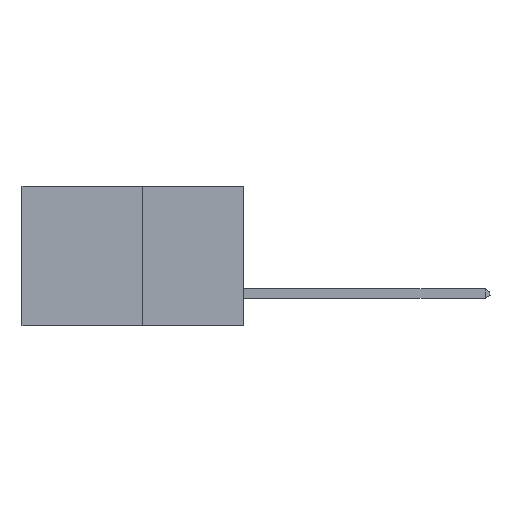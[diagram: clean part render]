
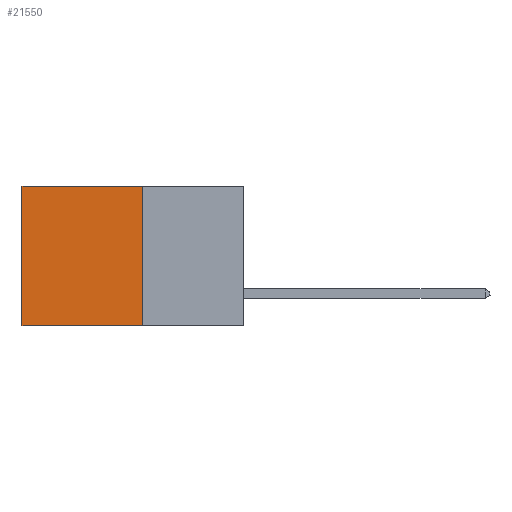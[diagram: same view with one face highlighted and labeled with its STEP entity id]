
A CAD part, left-side view. The second image highlights one B-rep face of the part: STEP entity #21550.
In plain terms, the highlighted planar face has unit normal (-1, 0, 0).
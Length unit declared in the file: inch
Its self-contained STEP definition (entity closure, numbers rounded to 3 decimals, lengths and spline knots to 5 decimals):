
#331 = DIRECTION ( 'NONE',  ( 1., 0., 0. ) ) ;
#1255 = VERTEX_POINT ( 'NONE', #13706 ) ;
#3681 = CARTESIAN_POINT ( 'NONE',  ( 0.277, 0.27, -0.37 ) ) ;
#4196 = VECTOR ( 'NONE', #21205, 39.37008 ) ;
#4664 = EDGE_CURVE ( 'NONE', #1255, #12371, #14679, .T. ) ;
#4812 = VECTOR ( 'NONE', #20931, 39.37008 ) ;
#6540 = FACE_OUTER_BOUND ( 'NONE', #20782, .T. ) ;
#7776 = EDGE_CURVE ( 'NONE', #10371, #21811, #14286, .T. ) ;
#7781 = ORIENTED_EDGE ( 'NONE', *, *, #18908, .T. ) ;
#8833 = PLANE ( 'NONE',  #16423 ) ;
#9362 = LINE ( 'NONE', #14276, #4812 ) ;
#9843 = CARTESIAN_POINT ( 'NONE',  ( 0.277, 0.59, -0.37 ) ) ;
#10187 = VECTOR ( 'NONE', #10879, 39.37008 ) ;
#10211 = ORIENTED_EDGE ( 'NONE', *, *, #17438, .F. ) ;
#10371 = VERTEX_POINT ( 'NONE', #11639 ) ;
#10879 = DIRECTION ( 'NONE',  ( 0., 1., 0. ) ) ;
#11639 = CARTESIAN_POINT ( 'NONE',  ( 0.277, 0.27, 0. ) ) ;
#12235 = DIRECTION ( 'NONE',  ( 0., 0., -1. ) ) ;
#12371 = VERTEX_POINT ( 'NONE', #9843 ) ;
#12611 = LINE ( 'NONE', #3681, #21577 ) ;
#13706 = CARTESIAN_POINT ( 'NONE',  ( 0.277, 0.27, -0.37 ) ) ;
#14099 = ORIENTED_EDGE ( 'NONE', *, *, #7776, .T. ) ;
#14276 = CARTESIAN_POINT ( 'NONE',  ( 0.277, 0.59, -0.37 ) ) ;
#14286 = LINE ( 'NONE', #19531, #4196 ) ;
#14659 = CARTESIAN_POINT ( 'NONE',  ( 0.277, 0.59, 0. ) ) ;
#14679 = LINE ( 'NONE', #19320, #10187 ) ;
#15496 = DIRECTION ( 'NONE',  ( 0., 0., -1. ) ) ;
#16423 = AXIS2_PLACEMENT_3D ( 'NONE', #20637, #331, #12235 ) ;
#17438 = EDGE_CURVE ( 'NONE', #10371, #1255, #12611, .T. ) ;
#18908 = EDGE_CURVE ( 'NONE', #21811, #12371, #9362, .T. ) ;
#19061 = ORIENTED_EDGE ( 'NONE', *, *, #4664, .F. ) ;
#19320 = CARTESIAN_POINT ( 'NONE',  ( 0.277, 0.27, -0.37 ) ) ;
#19531 = CARTESIAN_POINT ( 'NONE',  ( 0.277, 0.27, 0. ) ) ;
#20637 = CARTESIAN_POINT ( 'NONE',  ( 0.277, 0.27, -0.37 ) ) ;
#20782 = EDGE_LOOP ( 'NONE', ( #7781, #19061, #10211, #14099 ) ) ;
#20931 = DIRECTION ( 'NONE',  ( 0., 0., -1. ) ) ;
#21205 = DIRECTION ( 'NONE',  ( 0., 1., 0. ) ) ;
#21550 = ADVANCED_FACE ( 'NONE', ( #6540 ), #8833, .F. ) ;
#21577 = VECTOR ( 'NONE', #15496, 39.37008 ) ;
#21811 = VERTEX_POINT ( 'NONE', #14659 ) ;
